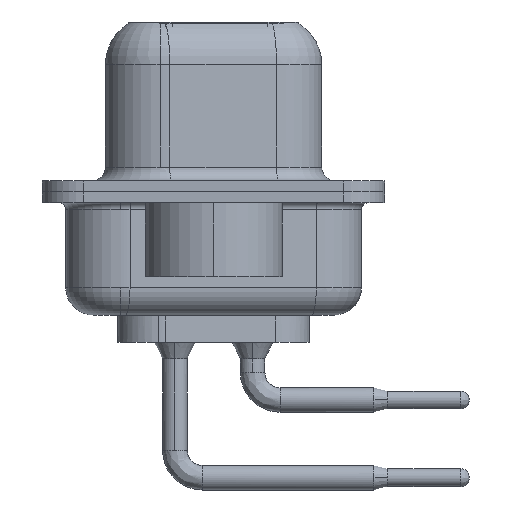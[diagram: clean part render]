
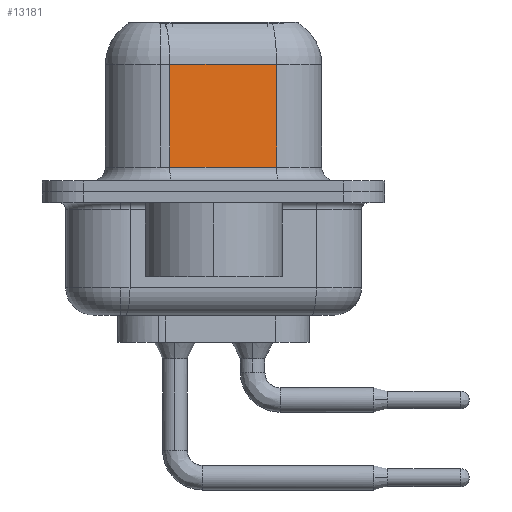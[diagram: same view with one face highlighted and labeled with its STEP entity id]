
A CAD part, left-side view. The second image highlights one B-rep face of the part: STEP entity #13181.
In plain terms, the highlighted planar face has unit normal (-0.985, -0.174, 0).
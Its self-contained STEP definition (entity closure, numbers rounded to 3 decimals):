
#1097 = CARTESIAN_POINT ( 'NONE',  ( 5.068, -2.297, 6.4 ) ) ;
#1823 = CARTESIAN_POINT ( 'NONE',  ( 5.068, -2.297, 0.9 ) ) ;
#2023 = DIRECTION ( 'NONE',  ( 0., 0., -1. ) ) ;
#2230 = LINE ( 'NONE', #12387, #5487 ) ;
#2547 = DIRECTION ( 'NONE',  ( -0.174, 0.985, 0. ) ) ;
#2712 = LINE ( 'NONE', #3452, #5926 ) ;
#3452 = CARTESIAN_POINT ( 'NONE',  ( 4.38, 1.603, 6.4 ) ) ;
#5222 = LINE ( 'NONE', #15827, #9317 ) ;
#5487 = VECTOR ( 'NONE', #9463, 1000. ) ;
#5812 = LINE ( 'NONE', #12491, #16549 ) ;
#5926 = VECTOR ( 'NONE', #2023, 1000. ) ;
#5940 = EDGE_LOOP ( 'NONE', ( #14470, #8594, #7659, #12349 ) ) ;
#6824 = DIRECTION ( 'NONE',  ( 0.174, -0.985, 0. ) ) ;
#7200 = CARTESIAN_POINT ( 'NONE',  ( 4.38, 1.603, 0.9 ) ) ;
#7313 = CARTESIAN_POINT ( 'NONE',  ( 4.38, 1.603, 4.65 ) ) ;
#7659 = ORIENTED_EDGE ( 'NONE', *, *, #16588, .T. ) ;
#8594 = ORIENTED_EDGE ( 'NONE', *, *, #12136, .T. ) ;
#9152 = EDGE_CURVE ( 'NONE', #10657, #14003, #2230, .T. ) ;
#9317 = VECTOR ( 'NONE', #17137, 1000. ) ;
#9463 = DIRECTION ( 'NONE',  ( 0., 0., -1. ) ) ;
#10657 = VERTEX_POINT ( 'NONE', #17870 ) ;
#10830 = PLANE ( 'NONE',  #13599 ) ;
#10890 = DIRECTION ( 'NONE',  ( 0.985, 0.174, 0. ) ) ;
#12136 = EDGE_CURVE ( 'NONE', #10657, #17106, #5222, .T. ) ;
#12349 = ORIENTED_EDGE ( 'NONE', *, *, #17865, .T. ) ;
#12387 = CARTESIAN_POINT ( 'NONE',  ( 5.068, -2.297, 6.4 ) ) ;
#12491 = CARTESIAN_POINT ( 'NONE',  ( 5.068, -2.297, 0.9 ) ) ;
#13181 = ADVANCED_FACE ( 'NONE', ( #14415 ), #10830, .F. ) ;
#13599 = AXIS2_PLACEMENT_3D ( 'NONE', #1097, #10890, #2547 ) ;
#13953 = VERTEX_POINT ( 'NONE', #7200 ) ;
#14003 = VERTEX_POINT ( 'NONE', #1823 ) ;
#14415 = FACE_OUTER_BOUND ( 'NONE', #5940, .T. ) ;
#14470 = ORIENTED_EDGE ( 'NONE', *, *, #9152, .F. ) ;
#15827 = CARTESIAN_POINT ( 'NONE',  ( 5.068, -2.297, 4.65 ) ) ;
#16549 = VECTOR ( 'NONE', #6824, 1000. ) ;
#16588 = EDGE_CURVE ( 'NONE', #17106, #13953, #2712, .T. ) ;
#17106 = VERTEX_POINT ( 'NONE', #7313 ) ;
#17137 = DIRECTION ( 'NONE',  ( -0.174, 0.985, 0. ) ) ;
#17865 = EDGE_CURVE ( 'NONE', #13953, #14003, #5812, .T. ) ;
#17870 = CARTESIAN_POINT ( 'NONE',  ( 5.068, -2.297, 4.65 ) ) ;
